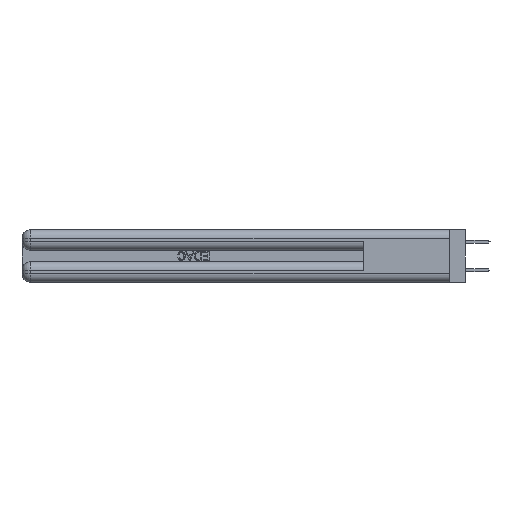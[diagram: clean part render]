
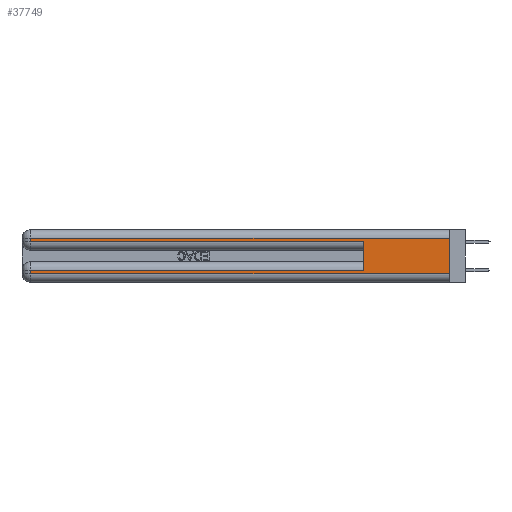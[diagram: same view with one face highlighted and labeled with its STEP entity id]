
A CAD part, left-side view. The second image highlights one B-rep face of the part: STEP entity #37749.
In plain terms, the highlighted planar face has unit normal (-1, 0, 0).
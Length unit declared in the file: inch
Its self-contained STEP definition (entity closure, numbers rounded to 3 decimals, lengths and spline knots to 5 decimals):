
#978 = CARTESIAN_POINT ( 'NONE',  ( 0., 2.94, 0.37 ) ) ;
#1180 = ORIENTED_EDGE ( 'NONE', *, *, #23521, .T. ) ;
#1737 = EDGE_CURVE ( 'NONE', #25419, #5181, #16503, .T. ) ;
#2024 = EDGE_CURVE ( 'NONE', #20728, #18128, #21084, .T. ) ;
#2094 = CARTESIAN_POINT ( 'NONE',  ( 0., 0., 0.06 ) ) ;
#2671 = VERTEX_POINT ( 'NONE', #46928 ) ;
#3179 = DIRECTION ( 'NONE',  ( 0., -1., 0. ) ) ;
#5181 = VERTEX_POINT ( 'NONE', #26965 ) ;
#5212 = CARTESIAN_POINT ( 'NONE',  ( 0., 0., 0.085 ) ) ;
#5537 = VECTOR ( 'NONE', #32485, 39.37008 ) ;
#6049 = EDGE_CURVE ( 'NONE', #17634, #18128, #38675, .T. ) ;
#6123 = ORIENTED_EDGE ( 'NONE', *, *, #6049, .F. ) ;
#6492 = VECTOR ( 'NONE', #31351, 39.37008 ) ;
#6540 = VECTOR ( 'NONE', #31680, 39.37008 ) ;
#6738 = ORIENTED_EDGE ( 'NONE', *, *, #22068, .F. ) ;
#6911 = CARTESIAN_POINT ( 'NONE',  ( 0., 0., 0.31 ) ) ;
#6967 = CARTESIAN_POINT ( 'NONE',  ( 0., 0., 0.37 ) ) ;
#8131 = VECTOR ( 'NONE', #34774, 39.37008 ) ;
#8807 = FACE_OUTER_BOUND ( 'NONE', #38554, .T. ) ;
#9309 = LINE ( 'NONE', #978, #28480 ) ;
#9548 = CARTESIAN_POINT ( 'NONE',  ( 0., 0., 0.31 ) ) ;
#10008 = VERTEX_POINT ( 'NONE', #27031 ) ;
#12200 = LINE ( 'NONE', #5212, #8131 ) ;
#14112 = LINE ( 'NONE', #34755, #6540 ) ;
#16347 = LINE ( 'NONE', #35262, #6492 ) ;
#16503 = LINE ( 'NONE', #32624, #36828 ) ;
#17624 = DIRECTION ( 'NONE',  ( 0., 1., 0. ) ) ;
#17634 = VERTEX_POINT ( 'NONE', #6911 ) ;
#18128 = VERTEX_POINT ( 'NONE', #2094 ) ;
#18229 = ORIENTED_EDGE ( 'NONE', *, *, #2024, .T. ) ;
#20728 = VERTEX_POINT ( 'NONE', #24265 ) ;
#21084 = LINE ( 'NONE', #22180, #26798 ) ;
#22068 = EDGE_CURVE ( 'NONE', #34014, #5181, #14112, .T. ) ;
#22180 = CARTESIAN_POINT ( 'NONE',  ( 0., 0., 0.06 ) ) ;
#22411 = EDGE_CURVE ( 'NONE', #10008, #20728, #16347, .T. ) ;
#22558 = CARTESIAN_POINT ( 'NONE',  ( 0., 0.6, 0.085 ) ) ;
#22980 = DIRECTION ( 'NONE',  ( 0., 0., -1. ) ) ;
#23521 = EDGE_CURVE ( 'NONE', #34014, #10008, #12200, .T. ) ;
#24265 = CARTESIAN_POINT ( 'NONE',  ( 0., 2.94, 0.06 ) ) ;
#24520 = DIRECTION ( 'NONE',  ( 0., 0., -1. ) ) ;
#25419 = VERTEX_POINT ( 'NONE', #45325 ) ;
#26798 = VECTOR ( 'NONE', #3179, 39.37008 ) ;
#26965 = CARTESIAN_POINT ( 'NONE',  ( 0., 0.6, 0.285 ) ) ;
#27031 = CARTESIAN_POINT ( 'NONE',  ( 0., 2.94, 0.085 ) ) ;
#28480 = VECTOR ( 'NONE', #22980, 39.37008 ) ;
#30282 = EDGE_CURVE ( 'NONE', #2671, #25419, #9309, .T. ) ;
#31351 = DIRECTION ( 'NONE',  ( 0., 0., -1. ) ) ;
#31680 = DIRECTION ( 'NONE',  ( 0., 0., 1. ) ) ;
#32381 = CARTESIAN_POINT ( 'NONE',  ( 0., 0., 0.37 ) ) ;
#32485 = DIRECTION ( 'NONE',  ( 0., 0., -1. ) ) ;
#32624 = CARTESIAN_POINT ( 'NONE',  ( 0., 0., 0.285 ) ) ;
#33074 = EDGE_CURVE ( 'NONE', #17634, #2671, #43525, .T. ) ;
#34014 = VERTEX_POINT ( 'NONE', #22558 ) ;
#34755 = CARTESIAN_POINT ( 'NONE',  ( 0., 0.6, 0.145 ) ) ;
#34774 = DIRECTION ( 'NONE',  ( 0., 1., 0. ) ) ;
#35019 = ORIENTED_EDGE ( 'NONE', *, *, #22411, .T. ) ;
#35262 = CARTESIAN_POINT ( 'NONE',  ( 0., 2.94, 0.37 ) ) ;
#36035 = DIRECTION ( 'NONE',  ( 0., -1., 0. ) ) ;
#36828 = VECTOR ( 'NONE', #36035, 39.37008 ) ;
#36887 = ORIENTED_EDGE ( 'NONE', *, *, #33074, .T. ) ;
#37749 = ADVANCED_FACE ( 'NONE', ( #8807 ), #43114, .F. ) ;
#38178 = AXIS2_PLACEMENT_3D ( 'NONE', #32381, #42781, #24520 ) ;
#38554 = EDGE_LOOP ( 'NONE', ( #6123, #36887, #45768, #43904, #6738, #1180, #35019, #18229 ) ) ;
#38675 = LINE ( 'NONE', #6967, #5537 ) ;
#38823 = VECTOR ( 'NONE', #17624, 39.37008 ) ;
#42781 = DIRECTION ( 'NONE',  ( 1., 0., 0. ) ) ;
#43114 = PLANE ( 'NONE',  #38178 ) ;
#43525 = LINE ( 'NONE', #9548, #38823 ) ;
#43904 = ORIENTED_EDGE ( 'NONE', *, *, #1737, .T. ) ;
#45325 = CARTESIAN_POINT ( 'NONE',  ( 0., 2.94, 0.285 ) ) ;
#45768 = ORIENTED_EDGE ( 'NONE', *, *, #30282, .T. ) ;
#46928 = CARTESIAN_POINT ( 'NONE',  ( 0., 2.94, 0.31 ) ) ;
